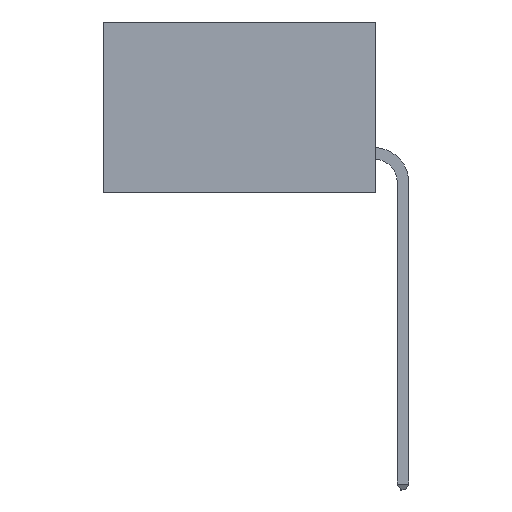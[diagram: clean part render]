
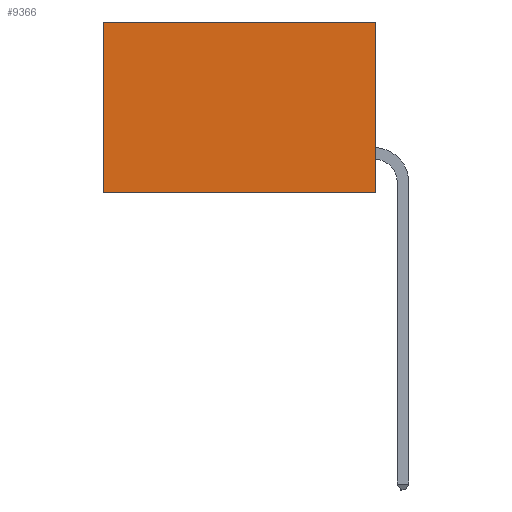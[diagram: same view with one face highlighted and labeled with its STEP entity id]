
A CAD part, left-side view. The second image highlights one B-rep face of the part: STEP entity #9366.
In plain terms, the highlighted planar face has unit normal (-1, 0, 0).
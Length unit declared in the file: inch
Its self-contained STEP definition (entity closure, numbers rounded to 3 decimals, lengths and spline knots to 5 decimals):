
#1400 = ORIENTED_EDGE ( 'NONE', *, *, #3845, .F. ) ;
#1638 = VECTOR ( 'NONE', #11303, 39.37008 ) ;
#1777 = VERTEX_POINT ( 'NONE', #5788 ) ;
#2608 = EDGE_CURVE ( 'NONE', #4764, #1777, #4108, .T. ) ;
#2836 = DIRECTION ( 'NONE',  ( 0., 1., 0. ) ) ;
#2934 = CARTESIAN_POINT ( 'NONE',  ( 0.277, 0., -0.37 ) ) ;
#2996 = CARTESIAN_POINT ( 'NONE',  ( 0.277, 0., -0.37 ) ) ;
#3291 = FACE_OUTER_BOUND ( 'NONE', #9680, .T. ) ;
#3608 = ORIENTED_EDGE ( 'NONE', *, *, #5951, .T. ) ;
#3845 = EDGE_CURVE ( 'NONE', #4764, #6894, #6469, .T. ) ;
#3867 = VECTOR ( 'NONE', #2836, 39.37008 ) ;
#3905 = VECTOR ( 'NONE', #7568, 39.37008 ) ;
#4108 = LINE ( 'NONE', #6173, #1638 ) ;
#4611 = DIRECTION ( 'NONE',  ( 1., 0., 0. ) ) ;
#4764 = VERTEX_POINT ( 'NONE', #5104 ) ;
#4768 = DIRECTION ( 'NONE',  ( 0., 0., -1. ) ) ;
#4864 = PLANE ( 'NONE',  #6483 ) ;
#5104 = CARTESIAN_POINT ( 'NONE',  ( 0.277, 0., 0. ) ) ;
#5149 = CARTESIAN_POINT ( 'NONE',  ( 0.277, 0., -0.37 ) ) ;
#5788 = CARTESIAN_POINT ( 'NONE',  ( 0.277, 0.59, 0. ) ) ;
#5951 = EDGE_CURVE ( 'NONE', #1777, #9642, #10625, .T. ) ;
#6173 = CARTESIAN_POINT ( 'NONE',  ( 0.277, 0., 0. ) ) ;
#6272 = ORIENTED_EDGE ( 'NONE', *, *, #2608, .T. ) ;
#6469 = LINE ( 'NONE', #9870, #10549 ) ;
#6483 = AXIS2_PLACEMENT_3D ( 'NONE', #5149, #4611, #4768 ) ;
#6894 = VERTEX_POINT ( 'NONE', #2934 ) ;
#7568 = DIRECTION ( 'NONE',  ( 0., 0., -1. ) ) ;
#7594 = CARTESIAN_POINT ( 'NONE',  ( 0.277, 0.59, -0.37 ) ) ;
#8828 = EDGE_CURVE ( 'NONE', #6894, #9642, #10353, .T. ) ;
#9366 = ADVANCED_FACE ( 'NONE', ( #3291 ), #4864, .F. ) ;
#9642 = VERTEX_POINT ( 'NONE', #10772 ) ;
#9680 = EDGE_LOOP ( 'NONE', ( #3608, #10378, #1400, #6272 ) ) ;
#9698 = DIRECTION ( 'NONE',  ( 0., 0., -1. ) ) ;
#9870 = CARTESIAN_POINT ( 'NONE',  ( 0.277, 0., -0.37 ) ) ;
#10353 = LINE ( 'NONE', #2996, #3867 ) ;
#10378 = ORIENTED_EDGE ( 'NONE', *, *, #8828, .F. ) ;
#10549 = VECTOR ( 'NONE', #9698, 39.37008 ) ;
#10625 = LINE ( 'NONE', #7594, #3905 ) ;
#10772 = CARTESIAN_POINT ( 'NONE',  ( 0.277, 0.59, -0.37 ) ) ;
#11303 = DIRECTION ( 'NONE',  ( 0., 1., 0. ) ) ;
